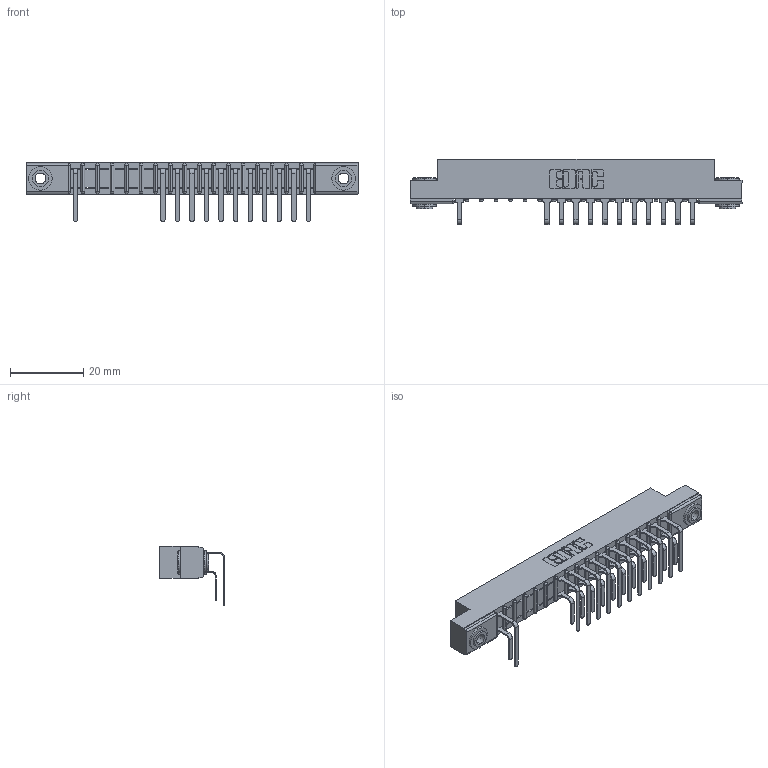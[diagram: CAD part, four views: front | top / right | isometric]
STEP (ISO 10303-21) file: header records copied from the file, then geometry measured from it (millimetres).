
FILE_DESCRIPTION (( 'STEP AP203' ), '1' );
FILE_NAME ('357-017-559-103.STEP', '2018-08-08T03:45:35', ( '' ), ( '' ), 'SwSTEP 2.0', 'SolidWorks 2016', '' );
FILE_SCHEMA (( 'CONFIG_CONTROL_DESIGN' ));
Length unit declared in the file: inch
Products named in the file (5): 357-017-559-103; 307 Part_.156 Dia Mounting Holes; 307-290-001_558 559 - 1 (Single); 307-290-001_559 - 2 (Single); 345-250-002_345-250-002-102
Assembly tree (27 placements, depth 2):
  357-017-559-103
    307 Part_.156 Dia Mounting Holes
    307-290-001_558 559 - 1 (Single)  x12
    307-290-001_559 - 2 (Single)  x12
    345-250-002_345-250-002-102  x2
Bounding box: 90.37 x 17.69 x 16.08 mm (x, y, z)
Volume: 5890.2 mm3; surface area: 10224.4 mm2
Topology: 27 solids, 27 shells, 1488 faces, 4163 edges, 2690 vertices
Faces by surface type: plane 946, cylinder 498, sphere 36, cone 8
Entity records: 20392 total; most frequent: CARTESIAN_POINT 3370, ORIENTED_EDGE 3338, DIRECTION 3315, EDGE_CURVE 1669, LINE 1261, VECTOR 1261, VERTEX_POINT 1082, AXIS2_PLACEMENT_3D 1027
